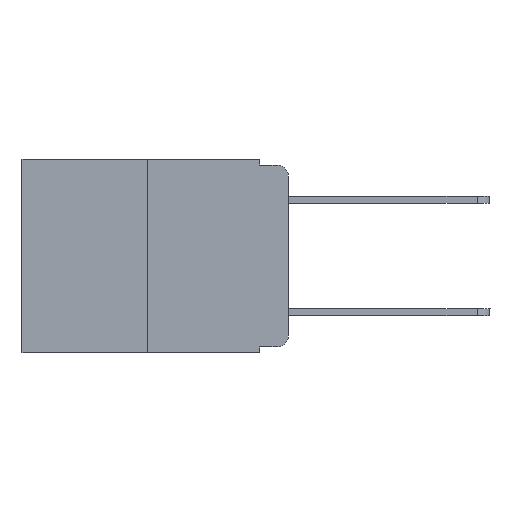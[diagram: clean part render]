
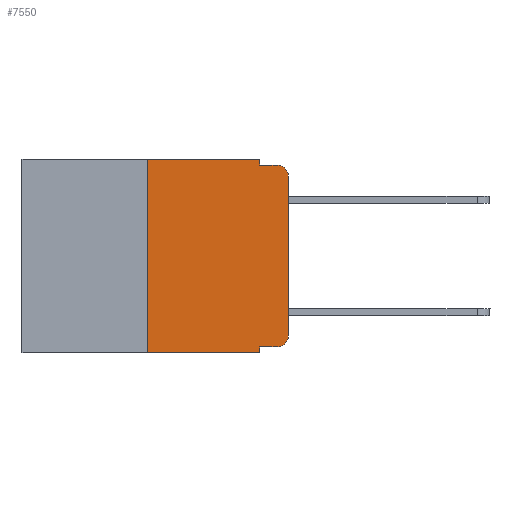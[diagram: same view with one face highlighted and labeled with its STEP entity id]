
A CAD part, left-side view. The second image highlights one B-rep face of the part: STEP entity #7550.
In plain terms, the highlighted planar face has unit normal (-1, 0, 0).
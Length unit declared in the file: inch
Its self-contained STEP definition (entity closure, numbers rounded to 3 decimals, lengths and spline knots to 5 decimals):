
#229 = DIRECTION ( 'NONE',  ( 0., 0., 1. ) ) ;
#304 = CARTESIAN_POINT ( 'NONE',  ( 0., 0.473, -0.343 ) ) ;
#433 = CARTESIAN_POINT ( 'NONE',  ( 0., 0., -0.03 ) ) ;
#668 = VERTEX_POINT ( 'NONE', #433 ) ;
#820 = VERTEX_POINT ( 'NONE', #12754 ) ;
#991 = CARTESIAN_POINT ( 'NONE',  ( 0., 0.051, -0.01 ) ) ;
#1146 = CIRCLE ( 'NONE', #3041, 0.02 ) ;
#1265 = AXIS2_PLACEMENT_3D ( 'NONE', #5713, #3765, #8453 ) ;
#1372 = ORIENTED_EDGE ( 'NONE', *, *, #5800, .F. ) ;
#1707 = DIRECTION ( 'NONE',  ( 0., 0., -1. ) ) ;
#1760 = CARTESIAN_POINT ( 'NONE',  ( 0., 0.051, 0. ) ) ;
#1783 = EDGE_CURVE ( 'NONE', #7094, #8862, #7265, .T. ) ;
#1811 = CARTESIAN_POINT ( 'NONE',  ( 0., 0.02, -0.313 ) ) ;
#2064 = DIRECTION ( 'NONE',  ( 0., -1., 0. ) ) ;
#2103 = CARTESIAN_POINT ( 'NONE',  ( 0., 0.25, 0. ) ) ;
#2315 = VECTOR ( 'NONE', #2064, 39.37008 ) ;
#2562 = ORIENTED_EDGE ( 'NONE', *, *, #3488, .T. ) ;
#2736 = LINE ( 'NONE', #9638, #6426 ) ;
#2882 = CARTESIAN_POINT ( 'NONE',  ( 0., 0.051, -0.343 ) ) ;
#2900 = DIRECTION ( 'NONE',  ( 0., -1., 0. ) ) ;
#2905 = EDGE_CURVE ( 'NONE', #668, #10462, #6948, .T. ) ;
#3041 = AXIS2_PLACEMENT_3D ( 'NONE', #1811, #6556, #8715 ) ;
#3331 = DIRECTION ( 'NONE',  ( 0., 0., -1. ) ) ;
#3488 = EDGE_CURVE ( 'NONE', #820, #668, #7256, .T. ) ;
#3562 = PLANE ( 'NONE',  #1265 ) ;
#3765 = DIRECTION ( 'NONE',  ( 1., 0., 0. ) ) ;
#3795 = ORIENTED_EDGE ( 'NONE', *, *, #1783, .T. ) ;
#3872 = LINE ( 'NONE', #991, #5474 ) ;
#3885 = EDGE_CURVE ( 'NONE', #7094, #5403, #5290, .T. ) ;
#4193 = DIRECTION ( 'NONE',  ( 0., 0., 1. ) ) ;
#4302 = VECTOR ( 'NONE', #229, 39.37008 ) ;
#4393 = ORIENTED_EDGE ( 'NONE', *, *, #9955, .F. ) ;
#4710 = ORIENTED_EDGE ( 'NONE', *, *, #9775, .F. ) ;
#5071 = VERTEX_POINT ( 'NONE', #8035 ) ;
#5150 = VERTEX_POINT ( 'NONE', #10051 ) ;
#5288 = EDGE_LOOP ( 'NONE', ( #2562, #6452, #4710, #4393, #5411, #7631, #3795, #1372, #8881, #10814 ) ) ;
#5290 = LINE ( 'NONE', #2103, #8268 ) ;
#5403 = VERTEX_POINT ( 'NONE', #6057 ) ;
#5411 = ORIENTED_EDGE ( 'NONE', *, *, #10667, .F. ) ;
#5474 = VECTOR ( 'NONE', #2900, 39.37008 ) ;
#5519 = VERTEX_POINT ( 'NONE', #7090 ) ;
#5614 = VERTEX_POINT ( 'NONE', #7283 ) ;
#5713 = CARTESIAN_POINT ( 'NONE',  ( 0., 0.473, 0. ) ) ;
#5800 = EDGE_CURVE ( 'NONE', #5614, #8862, #10654, .T. ) ;
#6057 = CARTESIAN_POINT ( 'NONE',  ( 0., 0.25, 0. ) ) ;
#6135 = AXIS2_PLACEMENT_3D ( 'NONE', #8735, #8799, #1707 ) ;
#6426 = VECTOR ( 'NONE', #12713, 39.37008 ) ;
#6452 = ORIENTED_EDGE ( 'NONE', *, *, #2905, .T. ) ;
#6513 = VECTOR ( 'NONE', #3331, 39.37008 ) ;
#6556 = DIRECTION ( 'NONE',  ( -1., 0., 0. ) ) ;
#6948 = CIRCLE ( 'NONE', #6135, 0.02 ) ;
#7046 = LINE ( 'NONE', #9140, #6513 ) ;
#7090 = CARTESIAN_POINT ( 'NONE',  ( 0., 0.051, 0. ) ) ;
#7094 = VERTEX_POINT ( 'NONE', #7438 ) ;
#7256 = LINE ( 'NONE', #10126, #4302 ) ;
#7265 = LINE ( 'NONE', #304, #2315 ) ;
#7283 = CARTESIAN_POINT ( 'NONE',  ( 0., 0.051, -0.333 ) ) ;
#7438 = CARTESIAN_POINT ( 'NONE',  ( 0., 0.25, -0.343 ) ) ;
#7550 = ADVANCED_FACE ( 'NONE', ( #12438 ), #3562, .F. ) ;
#7564 = VECTOR ( 'NONE', #9512, 39.37008 ) ;
#7631 = ORIENTED_EDGE ( 'NONE', *, *, #3885, .F. ) ;
#8035 = CARTESIAN_POINT ( 'NONE',  ( 0., 0.02, -0.333 ) ) ;
#8268 = VECTOR ( 'NONE', #4193, 39.37008 ) ;
#8453 = DIRECTION ( 'NONE',  ( 0., 0., -1. ) ) ;
#8715 = DIRECTION ( 'NONE',  ( 0., 0., -1. ) ) ;
#8735 = CARTESIAN_POINT ( 'NONE',  ( 0., 0.02, -0.03 ) ) ;
#8799 = DIRECTION ( 'NONE',  ( -1., 0., 0. ) ) ;
#8823 = VECTOR ( 'NONE', #12040, 39.37008 ) ;
#8862 = VERTEX_POINT ( 'NONE', #2882 ) ;
#8881 = ORIENTED_EDGE ( 'NONE', *, *, #9288, .T. ) ;
#8918 = CARTESIAN_POINT ( 'NONE',  ( 0., 0.473, 0. ) ) ;
#9110 = LINE ( 'NONE', #8918, #8823 ) ;
#9140 = CARTESIAN_POINT ( 'NONE',  ( 0., 0.051, 0. ) ) ;
#9288 = EDGE_CURVE ( 'NONE', #5614, #5071, #2736, .T. ) ;
#9512 = DIRECTION ( 'NONE',  ( 0., 0., -1. ) ) ;
#9638 = CARTESIAN_POINT ( 'NONE',  ( 0., 0.051, -0.333 ) ) ;
#9775 = EDGE_CURVE ( 'NONE', #5150, #10462, #3872, .T. ) ;
#9955 = EDGE_CURVE ( 'NONE', #5519, #5150, #7046, .T. ) ;
#10051 = CARTESIAN_POINT ( 'NONE',  ( 0., 0.051, -0.01 ) ) ;
#10126 = CARTESIAN_POINT ( 'NONE',  ( 0., 0., 0. ) ) ;
#10462 = VERTEX_POINT ( 'NONE', #11289 ) ;
#10654 = LINE ( 'NONE', #1760, #7564 ) ;
#10667 = EDGE_CURVE ( 'NONE', #5403, #5519, #9110, .T. ) ;
#10814 = ORIENTED_EDGE ( 'NONE', *, *, #12817, .T. ) ;
#11289 = CARTESIAN_POINT ( 'NONE',  ( 0., 0.02, -0.01 ) ) ;
#12040 = DIRECTION ( 'NONE',  ( 0., -1., 0. ) ) ;
#12438 = FACE_OUTER_BOUND ( 'NONE', #5288, .T. ) ;
#12713 = DIRECTION ( 'NONE',  ( 0., -1., 0. ) ) ;
#12754 = CARTESIAN_POINT ( 'NONE',  ( 0., 0., -0.313 ) ) ;
#12817 = EDGE_CURVE ( 'NONE', #5071, #820, #1146, .T. ) ;
